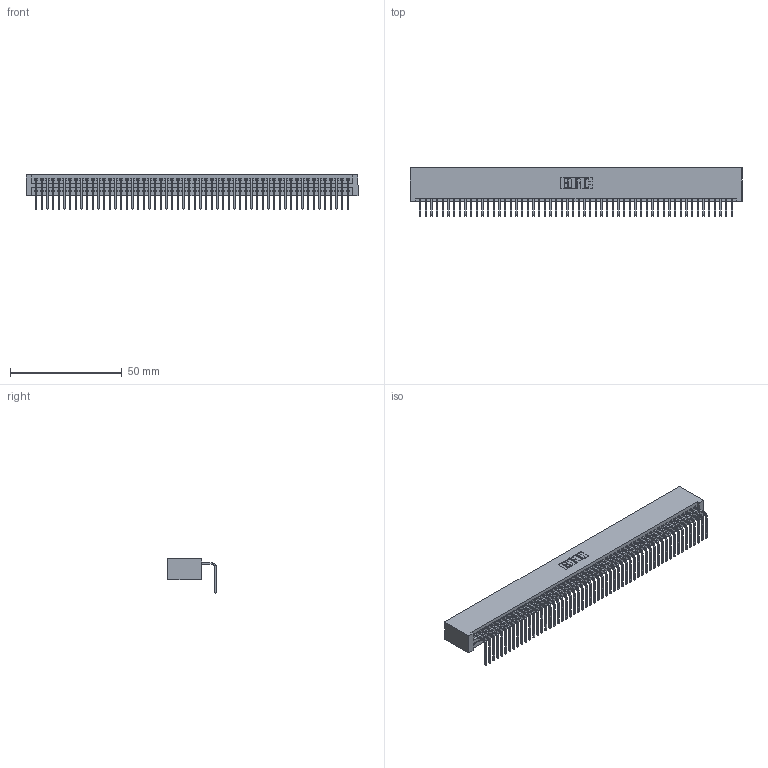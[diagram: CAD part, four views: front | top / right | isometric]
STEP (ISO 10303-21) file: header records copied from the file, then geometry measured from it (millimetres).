
FILE_DESCRIPTION (( 'STEP AP203' ), '1' );
FILE_NAME ('345-056-558-101.STEP', '2018-09-25T20:13:49', ( '' ), ( '' ), 'SwSTEP 2.0', 'SolidWorks 2016', '' );
FILE_SCHEMA (( 'CONFIG_CONTROL_DESIGN' ));
Length unit declared in the file: inch
Products named in the file (3): 345 Part_No Mounting Lugs; 345-056-558-101; 345-292-001_558 Tail - 2
Assembly tree (57 placements, depth 2):
  345-056-558-101
    345 Part_No Mounting Lugs
    345-292-001_558 Tail - 2  x56
Bounding box: 148.84 x 21.83 x 15.37 mm (x, y, z)
Volume: 15023 mm3; surface area: 21440.9 mm2
Topology: 57 solids, 57 shells, 3478 faces, 10509 edges, 6930 vertices
Faces by surface type: plane 2428, cylinder 1050
Entity records: 40069 total; most frequent: CARTESIAN_POINT 6948, ORIENTED_EDGE 6938, DIRECTION 6041, EDGE_CURVE 3469, LINE 3121, VECTOR 3121, VERTEX_POINT 2310, AXIS2_PLACEMENT_3D 1460
